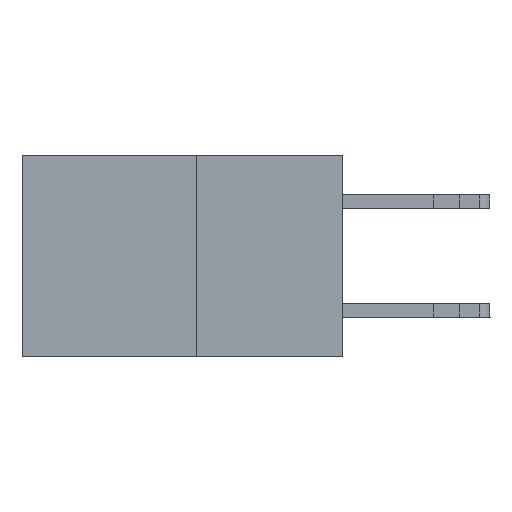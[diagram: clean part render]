
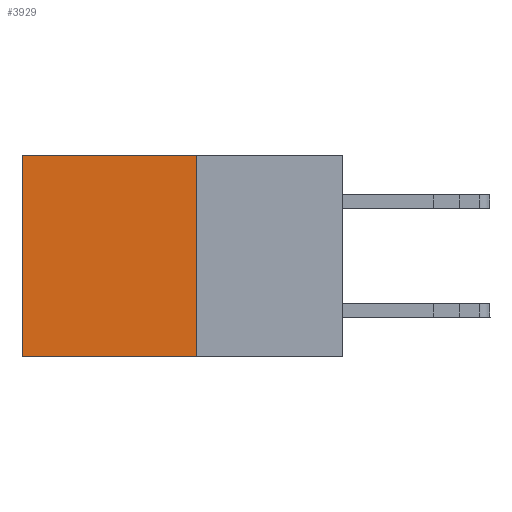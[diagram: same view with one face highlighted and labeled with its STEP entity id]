
A CAD part, left-side view. The second image highlights one B-rep face of the part: STEP entity #3929.
In plain terms, the highlighted planar face has unit normal (-1, 0, 0).
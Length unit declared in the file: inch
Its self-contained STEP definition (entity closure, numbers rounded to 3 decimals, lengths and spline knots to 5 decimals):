
#743 = VECTOR ( 'NONE', #10394, 39.37008 ) ;
#848 = CARTESIAN_POINT ( 'NONE',  ( 0.277, 0.27, -0.37 ) ) ;
#1246 = ORIENTED_EDGE ( 'NONE', *, *, #2596, .F. ) ;
#1608 = LINE ( 'NONE', #20171, #2947 ) ;
#2061 = EDGE_CURVE ( 'NONE', #17884, #23454, #7108, .T. ) ;
#2235 = CARTESIAN_POINT ( 'NONE',  ( 0.277, 0.59, -0.37 ) ) ;
#2596 = EDGE_CURVE ( 'NONE', #19825, #17700, #15679, .T. ) ;
#2808 = EDGE_LOOP ( 'NONE', ( #26226, #16092, #1246, #13438 ) ) ;
#2947 = VECTOR ( 'NONE', #9751, 39.37008 ) ;
#3650 = CARTESIAN_POINT ( 'NONE',  ( 0.277, 0.27, -0.37 ) ) ;
#3896 = DIRECTION ( 'NONE',  ( 1., 0., 0. ) ) ;
#3929 = ADVANCED_FACE ( 'NONE', ( #11309 ), #9242, .F. ) ;
#5132 = AXIS2_PLACEMENT_3D ( 'NONE', #3650, #3896, #14410 ) ;
#6278 = VECTOR ( 'NONE', #25647, 39.37008 ) ;
#6976 = CARTESIAN_POINT ( 'NONE',  ( 0.277, 0.27, 0. ) ) ;
#7108 = LINE ( 'NONE', #7390, #743 ) ;
#7390 = CARTESIAN_POINT ( 'NONE',  ( 0.277, 0.59, -0.37 ) ) ;
#9242 = PLANE ( 'NONE',  #5132 ) ;
#9751 = DIRECTION ( 'NONE',  ( 0., 1., 0. ) ) ;
#10310 = CARTESIAN_POINT ( 'NONE',  ( 0.277, 0.27, -0.37 ) ) ;
#10394 = DIRECTION ( 'NONE',  ( 0., 0., -1. ) ) ;
#10883 = CARTESIAN_POINT ( 'NONE',  ( 0.277, 0.59, 0. ) ) ;
#11309 = FACE_OUTER_BOUND ( 'NONE', #2808, .T. ) ;
#13438 = ORIENTED_EDGE ( 'NONE', *, *, #19434, .T. ) ;
#14410 = DIRECTION ( 'NONE',  ( 0., 0., -1. ) ) ;
#15679 = LINE ( 'NONE', #848, #25873 ) ;
#16092 = ORIENTED_EDGE ( 'NONE', *, *, #19619, .F. ) ;
#17700 = VERTEX_POINT ( 'NONE', #10310 ) ;
#17884 = VERTEX_POINT ( 'NONE', #10883 ) ;
#19434 = EDGE_CURVE ( 'NONE', #19825, #17884, #22934, .T. ) ;
#19619 = EDGE_CURVE ( 'NONE', #17700, #23454, #1608, .T. ) ;
#19825 = VERTEX_POINT ( 'NONE', #22737 ) ;
#20152 = DIRECTION ( 'NONE',  ( 0., 0., -1. ) ) ;
#20171 = CARTESIAN_POINT ( 'NONE',  ( 0.277, 0.27, -0.37 ) ) ;
#22737 = CARTESIAN_POINT ( 'NONE',  ( 0.277, 0.27, 0. ) ) ;
#22934 = LINE ( 'NONE', #6976, #6278 ) ;
#23454 = VERTEX_POINT ( 'NONE', #2235 ) ;
#25647 = DIRECTION ( 'NONE',  ( 0., 1., 0. ) ) ;
#25873 = VECTOR ( 'NONE', #20152, 39.37008 ) ;
#26226 = ORIENTED_EDGE ( 'NONE', *, *, #2061, .T. ) ;
